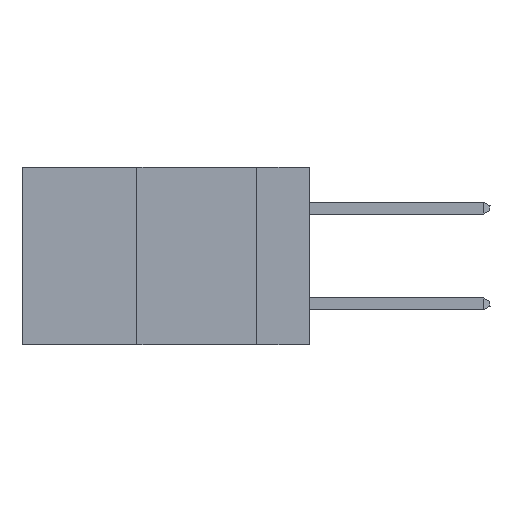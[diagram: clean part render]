
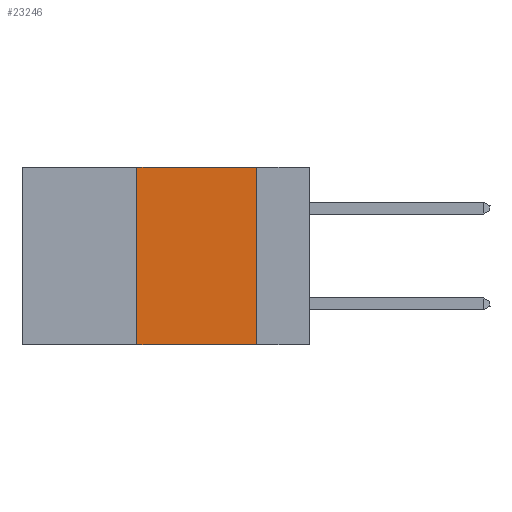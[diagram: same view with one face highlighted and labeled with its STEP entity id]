
A CAD part, left-side view. The second image highlights one B-rep face of the part: STEP entity #23246.
In plain terms, the highlighted planar face has unit normal (-1, 0, 0).
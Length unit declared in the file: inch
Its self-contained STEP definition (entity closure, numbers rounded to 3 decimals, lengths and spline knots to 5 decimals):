
#1342 = LINE ( 'NONE', #7150, #14960 ) ;
#1771 = CARTESIAN_POINT ( 'NONE',  ( 0., 0.11, -0.37 ) ) ;
#3988 = EDGE_LOOP ( 'NONE', ( #44459, #46520, #23446, #45189 ) ) ;
#4962 = VERTEX_POINT ( 'NONE', #5413 ) ;
#5413 = CARTESIAN_POINT ( 'NONE',  ( 0., 0.11, 0. ) ) ;
#6196 = CARTESIAN_POINT ( 'NONE',  ( 0., 0.36, -0.37 ) ) ;
#7150 = CARTESIAN_POINT ( 'NONE',  ( 0., 0.6, 0. ) ) ;
#7676 = EDGE_CURVE ( 'NONE', #4962, #33183, #28764, .T. ) ;
#8727 = LINE ( 'NONE', #31163, #34658 ) ;
#8776 = LINE ( 'NONE', #20783, #22346 ) ;
#9906 = DIRECTION ( 'NONE',  ( 0., 0., 1. ) ) ;
#12807 = CARTESIAN_POINT ( 'NONE',  ( 0., 0.11, 0. ) ) ;
#14007 = PLANE ( 'NONE',  #22991 ) ;
#14218 = EDGE_CURVE ( 'NONE', #28367, #33183, #8727, .T. ) ;
#14539 = DIRECTION ( 'NONE',  ( 0., -1., 0. ) ) ;
#14960 = VECTOR ( 'NONE', #14539, 39.37008 ) ;
#16858 = DIRECTION ( 'NONE',  ( 0., -1., 0. ) ) ;
#18412 = VERTEX_POINT ( 'NONE', #20002 ) ;
#20002 = CARTESIAN_POINT ( 'NONE',  ( 0., 0.36, 0. ) ) ;
#20783 = CARTESIAN_POINT ( 'NONE',  ( 0., 0.36, 0. ) ) ;
#22346 = VECTOR ( 'NONE', #9906, 39.37008 ) ;
#22615 = VECTOR ( 'NONE', #41083, 39.37008 ) ;
#22991 = AXIS2_PLACEMENT_3D ( 'NONE', #25553, #39243, #46700 ) ;
#23246 = ADVANCED_FACE ( 'NONE', ( #38106 ), #14007, .F. ) ;
#23446 = ORIENTED_EDGE ( 'NONE', *, *, #35672, .F. ) ;
#25553 = CARTESIAN_POINT ( 'NONE',  ( 0., 0.6, 0. ) ) ;
#28367 = VERTEX_POINT ( 'NONE', #6196 ) ;
#28764 = LINE ( 'NONE', #12807, #22615 ) ;
#31163 = CARTESIAN_POINT ( 'NONE',  ( 0., 0.6, -0.37 ) ) ;
#33183 = VERTEX_POINT ( 'NONE', #1771 ) ;
#34658 = VECTOR ( 'NONE', #16858, 39.37008 ) ;
#35672 = EDGE_CURVE ( 'NONE', #28367, #18412, #8776, .T. ) ;
#38106 = FACE_OUTER_BOUND ( 'NONE', #3988, .T. ) ;
#39243 = DIRECTION ( 'NONE',  ( 1., 0., 0. ) ) ;
#41083 = DIRECTION ( 'NONE',  ( 0., 0., -1. ) ) ;
#41803 = EDGE_CURVE ( 'NONE', #18412, #4962, #1342, .T. ) ;
#44459 = ORIENTED_EDGE ( 'NONE', *, *, #7676, .F. ) ;
#45189 = ORIENTED_EDGE ( 'NONE', *, *, #14218, .T. ) ;
#46520 = ORIENTED_EDGE ( 'NONE', *, *, #41803, .F. ) ;
#46700 = DIRECTION ( 'NONE',  ( 0., 0., -1. ) ) ;
